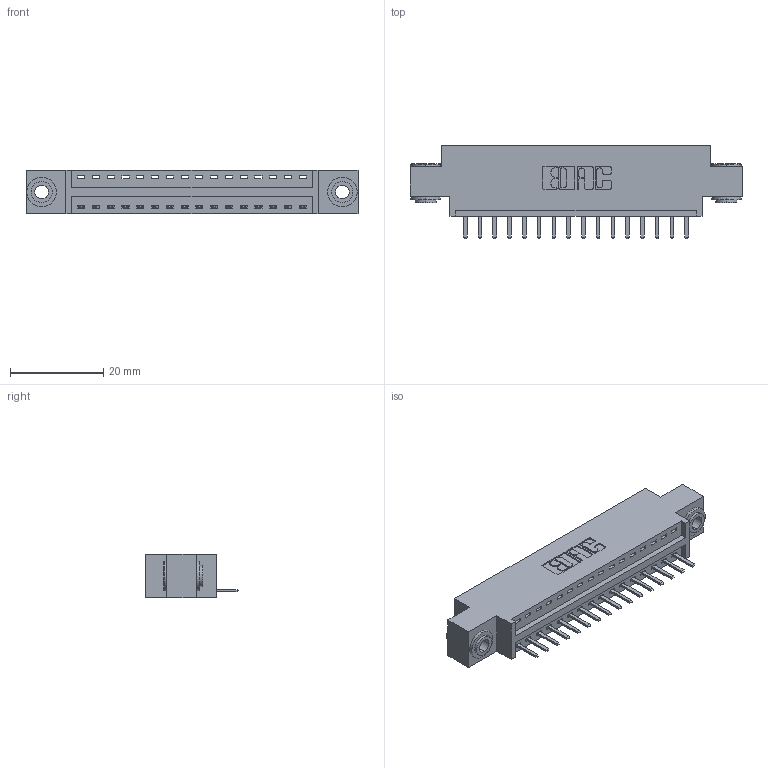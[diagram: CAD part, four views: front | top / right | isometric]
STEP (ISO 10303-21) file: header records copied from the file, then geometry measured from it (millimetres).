
FILE_DESCRIPTION (( 'STEP AP203' ), '1' );
FILE_NAME ('346-016-520-603.STEP', '2022-05-05T09:37:07', ( '' ), ( '' ), 'SwSTEP 2.0', 'SolidWorks 2020', '' );
FILE_SCHEMA (( 'CONFIG_CONTROL_DESIGN' ));
Length unit declared in the file: inch
Products named in the file (4): 345-292-001_345-293-120; 345-250-002_345-250-002-102; 346-016-520-603; 346 Part_0.170 Offset - 0.156 Dia-TH
Assembly tree (19 placements, depth 2):
  346-016-520-603
    346 Part_0.170 Offset - 0.156 Dia-TH
    345-292-001_345-293-120  x16
    345-250-002_345-250-002-102  x2
Bounding box: 71.37 x 20.02 x 9.4 mm (x, y, z)
Volume: 6453.6 mm3; surface area: 8043.8 mm2
Topology: 19 solids, 19 shells, 1170 faces, 3397 edges, 2218 vertices
Faces by surface type: plane 776, cylinder 386, cone 8
Entity records: 14742 total; most frequent: CARTESIAN_POINT 2529, ORIENTED_EDGE 2458, DIRECTION 2279, EDGE_CURVE 1229, LINE 1005, VECTOR 1005, VERTEX_POINT 814, AXIS2_PLACEMENT_3D 637
